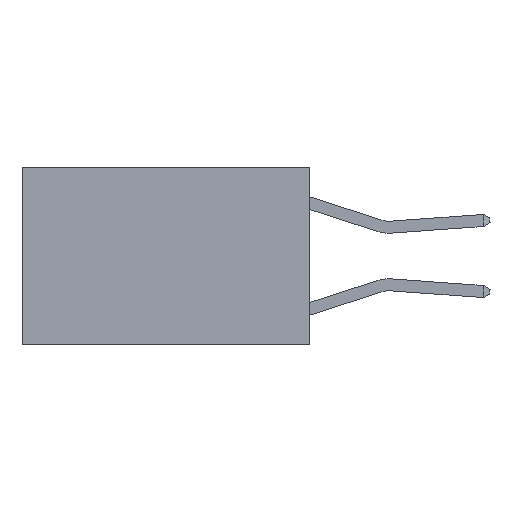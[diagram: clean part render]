
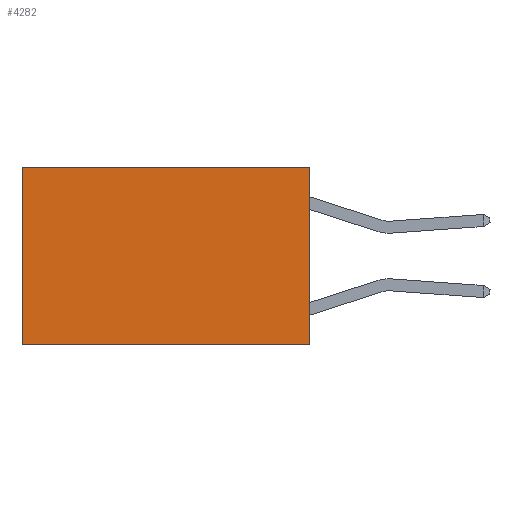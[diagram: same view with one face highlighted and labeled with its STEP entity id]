
A CAD part, left-side view. The second image highlights one B-rep face of the part: STEP entity #4282.
In plain terms, the highlighted planar face has unit normal (-1, 0, 0).
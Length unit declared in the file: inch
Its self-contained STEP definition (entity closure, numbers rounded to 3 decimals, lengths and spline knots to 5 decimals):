
#223 = FACE_OUTER_BOUND ( 'NONE', #816, .T. ) ;
#724 = ORIENTED_EDGE ( 'NONE', *, *, #7396, .F. ) ;
#794 = LINE ( 'NONE', #8445, #5865 ) ;
#816 = EDGE_LOOP ( 'NONE', ( #9354, #724, #3091, #2862 ) ) ;
#1312 = VERTEX_POINT ( 'NONE', #8032 ) ;
#1726 = DIRECTION ( 'NONE',  ( 0., 0., -1. ) ) ;
#2082 = EDGE_CURVE ( 'NONE', #4227, #7234, #6002, .T. ) ;
#2242 = LINE ( 'NONE', #12368, #6513 ) ;
#2527 = AXIS2_PLACEMENT_3D ( 'NONE', #10356, #7046, #13741 ) ;
#2563 = LINE ( 'NONE', #13806, #8006 ) ;
#2862 = ORIENTED_EDGE ( 'NONE', *, *, #12770, .T. ) ;
#3073 = VERTEX_POINT ( 'NONE', #10332 ) ;
#3091 = ORIENTED_EDGE ( 'NONE', *, *, #11072, .F. ) ;
#3518 = VECTOR ( 'NONE', #4928, 39.37008 ) ;
#4227 = VERTEX_POINT ( 'NONE', #13521 ) ;
#4282 = ADVANCED_FACE ( 'NONE', ( #223 ), #12580, .F. ) ;
#4887 = DIRECTION ( 'NONE',  ( 0., 1., 0. ) ) ;
#4928 = DIRECTION ( 'NONE',  ( 0., 0., -1. ) ) ;
#5627 = DIRECTION ( 'NONE',  ( 0., 1., 0. ) ) ;
#5865 = VECTOR ( 'NONE', #1726, 39.37008 ) ;
#6002 = LINE ( 'NONE', #12689, #3518 ) ;
#6513 = VECTOR ( 'NONE', #5627, 39.37008 ) ;
#7046 = DIRECTION ( 'NONE',  ( 1., 0., 0. ) ) ;
#7234 = VERTEX_POINT ( 'NONE', #9858 ) ;
#7396 = EDGE_CURVE ( 'NONE', #3073, #7234, #2242, .T. ) ;
#8006 = VECTOR ( 'NONE', #4887, 39.37008 ) ;
#8032 = CARTESIAN_POINT ( 'NONE',  ( 0.2625, 0., 0. ) ) ;
#8445 = CARTESIAN_POINT ( 'NONE',  ( 0.2625, 0., 0. ) ) ;
#9354 = ORIENTED_EDGE ( 'NONE', *, *, #2082, .T. ) ;
#9858 = CARTESIAN_POINT ( 'NONE',  ( 0.2625, 0.6, -0.37 ) ) ;
#10332 = CARTESIAN_POINT ( 'NONE',  ( 0.2625, 0., -0.37 ) ) ;
#10356 = CARTESIAN_POINT ( 'NONE',  ( 0.2625, 0., 0. ) ) ;
#11072 = EDGE_CURVE ( 'NONE', #1312, #3073, #794, .T. ) ;
#12368 = CARTESIAN_POINT ( 'NONE',  ( 0.2625, 0., -0.37 ) ) ;
#12580 = PLANE ( 'NONE',  #2527 ) ;
#12689 = CARTESIAN_POINT ( 'NONE',  ( 0.2625, 0.6, 0. ) ) ;
#12770 = EDGE_CURVE ( 'NONE', #1312, #4227, #2563, .T. ) ;
#13521 = CARTESIAN_POINT ( 'NONE',  ( 0.2625, 0.6, 0. ) ) ;
#13741 = DIRECTION ( 'NONE',  ( 0., 0., -1. ) ) ;
#13806 = CARTESIAN_POINT ( 'NONE',  ( 0.2625, 0., 0. ) ) ;
